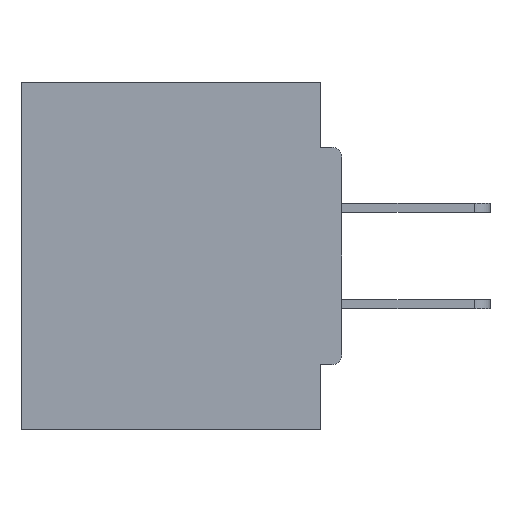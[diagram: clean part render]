
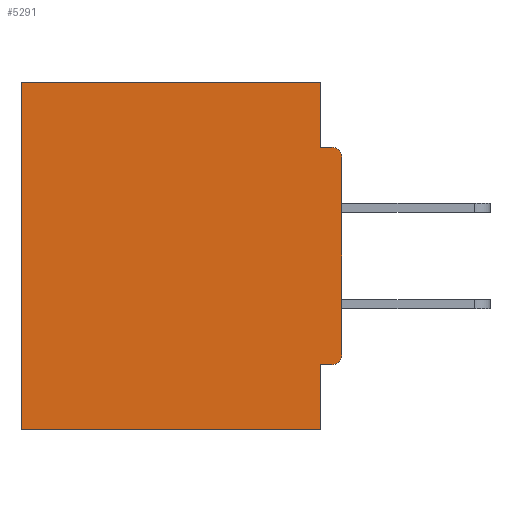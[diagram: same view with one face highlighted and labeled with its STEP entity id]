
A CAD part, left-side view. The second image highlights one B-rep face of the part: STEP entity #5291.
In plain terms, the highlighted planar face has unit normal (-1, 0, 0).
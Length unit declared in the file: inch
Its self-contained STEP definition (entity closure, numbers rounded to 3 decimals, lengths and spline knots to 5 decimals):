
#635 = EDGE_CURVE ( 'NONE', #26444, #17656, #6803, .T. ) ;
#1338 = EDGE_CURVE ( 'NONE', #25283, #26444, #21453, .T. ) ;
#2132 = DIRECTION ( 'NONE',  ( 0., 1., 0. ) ) ;
#2323 = PLANE ( 'NONE',  #19516 ) ;
#3668 = CARTESIAN_POINT ( 'NONE',  ( 0.298, 0.031, -0.0935 ) ) ;
#3942 = LINE ( 'NONE', #9180, #16757 ) ;
#4029 = VECTOR ( 'NONE', #39324, 39.37008 ) ;
#4854 = CARTESIAN_POINT ( 'NONE',  ( 0.298, 0.46, 0. ) ) ;
#4944 = VERTEX_POINT ( 'NONE', #24490 ) ;
#5179 = LINE ( 'NONE', #34807, #36523 ) ;
#5291 = ADVANCED_FACE ( 'NONE', ( #28901 ), #2323, .F. ) ;
#6314 = EDGE_CURVE ( 'NONE', #8423, #13781, #20272, .T. ) ;
#6803 = LINE ( 'NONE', #4854, #38090 ) ;
#7178 = VECTOR ( 'NONE', #2132, 39.37008 ) ;
#7936 = AXIS2_PLACEMENT_3D ( 'NONE', #14584, #29911, #26959 ) ;
#8423 = VERTEX_POINT ( 'NONE', #34154 ) ;
#9180 = CARTESIAN_POINT ( 'NONE',  ( 0.298, 0., -0.5 ) ) ;
#10589 = VERTEX_POINT ( 'NONE', #3668 ) ;
#11012 = CARTESIAN_POINT ( 'NONE',  ( 0.298, 0.031, 0. ) ) ;
#11428 = CARTESIAN_POINT ( 'NONE',  ( 0.298, 0., -0.3915 ) ) ;
#11700 = VECTOR ( 'NONE', #22586, 39.37008 ) ;
#11720 = VERTEX_POINT ( 'NONE', #33962 ) ;
#12155 = EDGE_CURVE ( 'NONE', #8423, #4944, #12800, .T. ) ;
#12370 = DIRECTION ( 'NONE',  ( 0., 1., 0. ) ) ;
#12800 = CIRCLE ( 'NONE', #37801, 0.015 ) ;
#13255 = DIRECTION ( 'NONE',  ( -1., 0., 0. ) ) ;
#13781 = VERTEX_POINT ( 'NONE', #11428 ) ;
#14521 = VERTEX_POINT ( 'NONE', #14945 ) ;
#14584 = CARTESIAN_POINT ( 'NONE',  ( 0.298, 0.015, -0.3915 ) ) ;
#14768 = DIRECTION ( 'NONE',  ( 1., 0., 0. ) ) ;
#14945 = CARTESIAN_POINT ( 'NONE',  ( 0.298, 0.031, -0.4065 ) ) ;
#15589 = EDGE_CURVE ( 'NONE', #10589, #4944, #20156, .T. ) ;
#16309 = DIRECTION ( 'NONE',  ( 0., 0., -1. ) ) ;
#16611 = DIRECTION ( 'NONE',  ( 0., 0., -1. ) ) ;
#16757 = VECTOR ( 'NONE', #12370, 39.37008 ) ;
#17011 = ORIENTED_EDGE ( 'NONE', *, *, #29541, .F. ) ;
#17049 = EDGE_CURVE ( 'NONE', #11720, #14521, #37036, .T. ) ;
#17266 = ORIENTED_EDGE ( 'NONE', *, *, #27264, .T. ) ;
#17656 = VERTEX_POINT ( 'NONE', #21899 ) ;
#18109 = CIRCLE ( 'NONE', #7936, 0.015 ) ;
#19516 = AXIS2_PLACEMENT_3D ( 'NONE', #26882, #14768, #29957 ) ;
#19917 = ORIENTED_EDGE ( 'NONE', *, *, #12155, .T. ) ;
#20156 = LINE ( 'NONE', #21030, #4029 ) ;
#20272 = LINE ( 'NONE', #38047, #11700 ) ;
#20801 = LINE ( 'NONE', #26443, #25101 ) ;
#21030 = CARTESIAN_POINT ( 'NONE',  ( 0.298, 0., -0.0935 ) ) ;
#21123 = ORIENTED_EDGE ( 'NONE', *, *, #17049, .F. ) ;
#21453 = LINE ( 'NONE', #23950, #32833 ) ;
#21899 = CARTESIAN_POINT ( 'NONE',  ( 0.298, 0.46, -0.5 ) ) ;
#22586 = DIRECTION ( 'NONE',  ( 0., 0., -1. ) ) ;
#22839 = CARTESIAN_POINT ( 'NONE',  ( 0.298, 0.015, -0.1085 ) ) ;
#22953 = ORIENTED_EDGE ( 'NONE', *, *, #15589, .F. ) ;
#23830 = EDGE_CURVE ( 'NONE', #14521, #23909, #20801, .T. ) ;
#23909 = VERTEX_POINT ( 'NONE', #32947 ) ;
#23950 = CARTESIAN_POINT ( 'NONE',  ( 0.298, 0., 0. ) ) ;
#24490 = CARTESIAN_POINT ( 'NONE',  ( 0.298, 0.015, -0.0935 ) ) ;
#24692 = ORIENTED_EDGE ( 'NONE', *, *, #26286, .F. ) ;
#25101 = VECTOR ( 'NONE', #32557, 39.37008 ) ;
#25151 = CARTESIAN_POINT ( 'NONE',  ( 0.298, 0.46, 0. ) ) ;
#25283 = VERTEX_POINT ( 'NONE', #11012 ) ;
#25960 = DIRECTION ( 'NONE',  ( 0., 0., -1. ) ) ;
#26286 = EDGE_CURVE ( 'NONE', #23909, #17656, #3942, .T. ) ;
#26443 = CARTESIAN_POINT ( 'NONE',  ( 0.298, 0.031, -0.5 ) ) ;
#26444 = VERTEX_POINT ( 'NONE', #25151 ) ;
#26882 = CARTESIAN_POINT ( 'NONE',  ( 0.298, 0., 0. ) ) ;
#26959 = DIRECTION ( 'NONE',  ( 0., 0., -1. ) ) ;
#26978 = DIRECTION ( 'NONE',  ( 0., 1., 0. ) ) ;
#27264 = EDGE_CURVE ( 'NONE', #11720, #13781, #18109, .T. ) ;
#28901 = FACE_OUTER_BOUND ( 'NONE', #34084, .T. ) ;
#29541 = EDGE_CURVE ( 'NONE', #25283, #10589, #5179, .T. ) ;
#29604 = ORIENTED_EDGE ( 'NONE', *, *, #635, .T. ) ;
#29911 = DIRECTION ( 'NONE',  ( -1., 0., 0. ) ) ;
#29957 = DIRECTION ( 'NONE',  ( 0., 0., -1. ) ) ;
#30090 = ORIENTED_EDGE ( 'NONE', *, *, #6314, .F. ) ;
#32403 = CARTESIAN_POINT ( 'NONE',  ( 0.298, 0., -0.4065 ) ) ;
#32557 = DIRECTION ( 'NONE',  ( 0., 0., -1. ) ) ;
#32833 = VECTOR ( 'NONE', #26978, 39.37008 ) ;
#32947 = CARTESIAN_POINT ( 'NONE',  ( 0.298, 0.031, -0.5 ) ) ;
#33515 = ORIENTED_EDGE ( 'NONE', *, *, #1338, .T. ) ;
#33847 = ORIENTED_EDGE ( 'NONE', *, *, #23830, .F. ) ;
#33962 = CARTESIAN_POINT ( 'NONE',  ( 0.298, 0.015, -0.4065 ) ) ;
#34084 = EDGE_LOOP ( 'NONE', ( #19917, #22953, #17011, #33515, #29604, #24692, #33847, #21123, #17266, #30090 ) ) ;
#34154 = CARTESIAN_POINT ( 'NONE',  ( 0.298, 0., -0.1085 ) ) ;
#34807 = CARTESIAN_POINT ( 'NONE',  ( 0.298, 0.031, -0.5 ) ) ;
#36523 = VECTOR ( 'NONE', #16611, 39.37008 ) ;
#37036 = LINE ( 'NONE', #32403, #7178 ) ;
#37801 = AXIS2_PLACEMENT_3D ( 'NONE', #22839, #13255, #16309 ) ;
#38047 = CARTESIAN_POINT ( 'NONE',  ( 0.298, 0., 0. ) ) ;
#38090 = VECTOR ( 'NONE', #25960, 39.37008 ) ;
#39324 = DIRECTION ( 'NONE',  ( 0., -1., 0. ) ) ;
